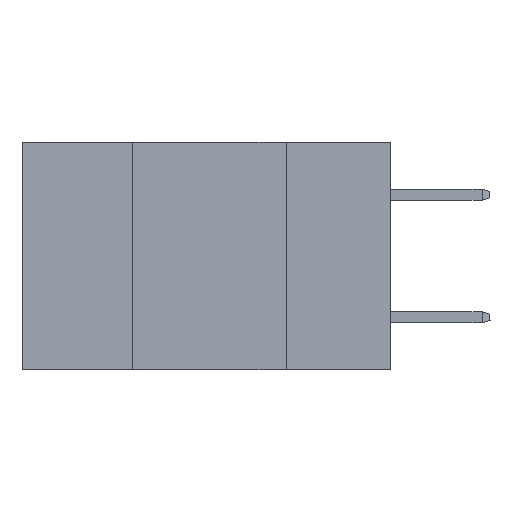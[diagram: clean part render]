
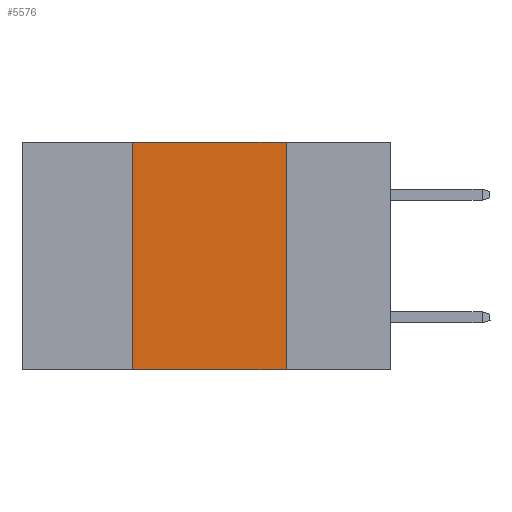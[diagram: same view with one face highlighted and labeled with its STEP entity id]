
A CAD part, left-side view. The second image highlights one B-rep face of the part: STEP entity #5576.
In plain terms, the highlighted planar face has unit normal (-1, 0, 0).
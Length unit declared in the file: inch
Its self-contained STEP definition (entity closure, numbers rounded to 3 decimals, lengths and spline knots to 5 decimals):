
#2817 = CARTESIAN_POINT ( 'NONE',  ( 0., 0.17, 0. ) ) ;
#2833 = CARTESIAN_POINT ( 'NONE',  ( 0., 0.17, 0. ) ) ;
#3125 = VERTEX_POINT ( 'NONE', #13626 ) ;
#3389 = CARTESIAN_POINT ( 'NONE',  ( 0., 0.6, 0. ) ) ;
#4024 = CARTESIAN_POINT ( 'NONE',  ( 0., 0.17, -0.37 ) ) ;
#5576 = ADVANCED_FACE ( 'NONE', ( #6730 ), #10404, .F. ) ;
#6007 = DIRECTION ( 'NONE',  ( 0., 0., -1. ) ) ;
#6189 = VERTEX_POINT ( 'NONE', #2833 ) ;
#6434 = LINE ( 'NONE', #14972, #18518 ) ;
#6730 = FACE_OUTER_BOUND ( 'NONE', #7390, .T. ) ;
#6855 = DIRECTION ( 'NONE',  ( 0., -1., 0. ) ) ;
#6892 = EDGE_CURVE ( 'NONE', #3125, #6189, #6434, .T. ) ;
#7390 = EDGE_LOOP ( 'NONE', ( #11236, #16080, #14609, #7869 ) ) ;
#7869 = ORIENTED_EDGE ( 'NONE', *, *, #16902, .T. ) ;
#8956 = CARTESIAN_POINT ( 'NONE',  ( 0., 0.42, 0. ) ) ;
#9892 = DIRECTION ( 'NONE',  ( 0., -1., 0. ) ) ;
#9922 = VECTOR ( 'NONE', #6855, 39.37008 ) ;
#10404 = PLANE ( 'NONE',  #18674 ) ;
#11236 = ORIENTED_EDGE ( 'NONE', *, *, #20860, .F. ) ;
#11768 = VECTOR ( 'NONE', #14187, 39.37008 ) ;
#12453 = CARTESIAN_POINT ( 'NONE',  ( 0., 0.42, -0.37 ) ) ;
#12515 = VERTEX_POINT ( 'NONE', #4024 ) ;
#12864 = LINE ( 'NONE', #8956, #11768 ) ;
#13626 = CARTESIAN_POINT ( 'NONE',  ( 0., 0.42, 0. ) ) ;
#13880 = CARTESIAN_POINT ( 'NONE',  ( 0., 0.6, -0.37 ) ) ;
#14187 = DIRECTION ( 'NONE',  ( 0., 0., 1. ) ) ;
#14609 = ORIENTED_EDGE ( 'NONE', *, *, #21981, .F. ) ;
#14972 = CARTESIAN_POINT ( 'NONE',  ( 0., 0.6, 0. ) ) ;
#15369 = DIRECTION ( 'NONE',  ( 1., 0., 0. ) ) ;
#16072 = LINE ( 'NONE', #13880, #9922 ) ;
#16080 = ORIENTED_EDGE ( 'NONE', *, *, #6892, .F. ) ;
#16736 = VECTOR ( 'NONE', #6007, 39.37008 ) ;
#16902 = EDGE_CURVE ( 'NONE', #18066, #12515, #16072, .T. ) ;
#17292 = DIRECTION ( 'NONE',  ( 0., 0., -1. ) ) ;
#18066 = VERTEX_POINT ( 'NONE', #12453 ) ;
#18518 = VECTOR ( 'NONE', #9892, 39.37008 ) ;
#18674 = AXIS2_PLACEMENT_3D ( 'NONE', #3389, #15369, #17292 ) ;
#18894 = LINE ( 'NONE', #2817, #16736 ) ;
#20860 = EDGE_CURVE ( 'NONE', #6189, #12515, #18894, .T. ) ;
#21981 = EDGE_CURVE ( 'NONE', #18066, #3125, #12864, .T. ) ;
